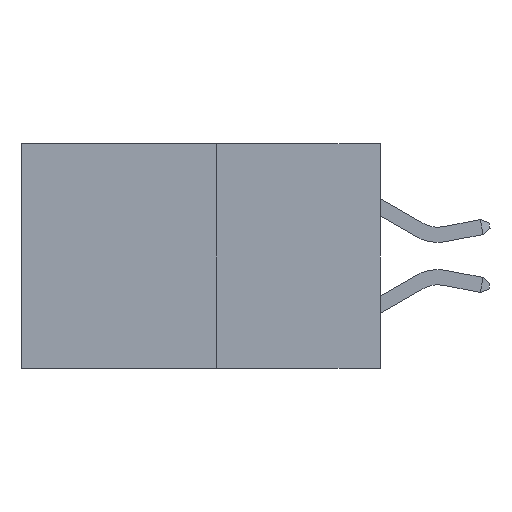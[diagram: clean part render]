
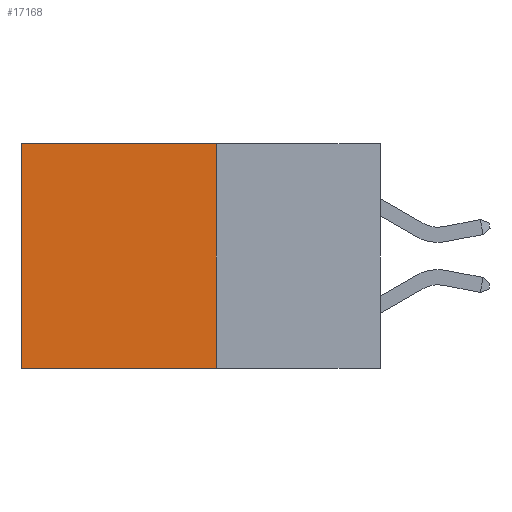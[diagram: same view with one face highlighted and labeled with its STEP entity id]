
A CAD part, left-side view. The second image highlights one B-rep face of the part: STEP entity #17168.
In plain terms, the highlighted planar face has unit normal (-1, 0, 0).
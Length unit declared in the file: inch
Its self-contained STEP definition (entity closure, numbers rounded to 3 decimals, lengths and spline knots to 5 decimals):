
#530 = CARTESIAN_POINT ( 'NONE',  ( 0.277, 0.27, 0. ) ) ;
#603 = ORIENTED_EDGE ( 'NONE', *, *, #21764, .T. ) ;
#740 = CARTESIAN_POINT ( 'NONE',  ( 0.277, 0.27, -0.37 ) ) ;
#845 = AXIS2_PLACEMENT_3D ( 'NONE', #16430, #6178, #18108 ) ;
#2040 = VERTEX_POINT ( 'NONE', #20734 ) ;
#2538 = DIRECTION ( 'NONE',  ( 0., 0., -1. ) ) ;
#3259 = VERTEX_POINT ( 'NONE', #20057 ) ;
#4427 = PLANE ( 'NONE',  #845 ) ;
#4671 = VECTOR ( 'NONE', #7100, 39.37008 ) ;
#4833 = ORIENTED_EDGE ( 'NONE', *, *, #20428, .F. ) ;
#4965 = EDGE_LOOP ( 'NONE', ( #603, #4833, #15438, #12558 ) ) ;
#5117 = VERTEX_POINT ( 'NONE', #6307 ) ;
#5258 = CARTESIAN_POINT ( 'NONE',  ( 0.277, 0.27, -0.37 ) ) ;
#6178 = DIRECTION ( 'NONE',  ( 1., 0., 0. ) ) ;
#6307 = CARTESIAN_POINT ( 'NONE',  ( 0.277, 0.59, 0. ) ) ;
#6370 = VECTOR ( 'NONE', #12869, 39.37008 ) ;
#7100 = DIRECTION ( 'NONE',  ( 0., 0., -1. ) ) ;
#7269 = VERTEX_POINT ( 'NONE', #16856 ) ;
#9261 = LINE ( 'NONE', #5258, #4671 ) ;
#9419 = CARTESIAN_POINT ( 'NONE',  ( 0.277, 0.59, -0.37 ) ) ;
#10542 = VECTOR ( 'NONE', #14368, 39.37008 ) ;
#10627 = EDGE_CURVE ( 'NONE', #2040, #7269, #9261, .T. ) ;
#12558 = ORIENTED_EDGE ( 'NONE', *, *, #12664, .T. ) ;
#12664 = EDGE_CURVE ( 'NONE', #2040, #5117, #13997, .T. ) ;
#12869 = DIRECTION ( 'NONE',  ( 0., 1., 0. ) ) ;
#13317 = VECTOR ( 'NONE', #2538, 39.37008 ) ;
#13997 = LINE ( 'NONE', #530, #10542 ) ;
#14001 = FACE_OUTER_BOUND ( 'NONE', #4965, .T. ) ;
#14368 = DIRECTION ( 'NONE',  ( 0., 1., 0. ) ) ;
#15438 = ORIENTED_EDGE ( 'NONE', *, *, #10627, .F. ) ;
#16430 = CARTESIAN_POINT ( 'NONE',  ( 0.277, 0.27, -0.37 ) ) ;
#16856 = CARTESIAN_POINT ( 'NONE',  ( 0.277, 0.27, -0.37 ) ) ;
#17168 = ADVANCED_FACE ( 'NONE', ( #14001 ), #4427, .F. ) ;
#17765 = LINE ( 'NONE', #9419, #13317 ) ;
#18108 = DIRECTION ( 'NONE',  ( 0., 0., -1. ) ) ;
#19395 = LINE ( 'NONE', #740, #6370 ) ;
#20057 = CARTESIAN_POINT ( 'NONE',  ( 0.277, 0.59, -0.37 ) ) ;
#20428 = EDGE_CURVE ( 'NONE', #7269, #3259, #19395, .T. ) ;
#20734 = CARTESIAN_POINT ( 'NONE',  ( 0.277, 0.27, 0. ) ) ;
#21764 = EDGE_CURVE ( 'NONE', #5117, #3259, #17765, .T. ) ;
